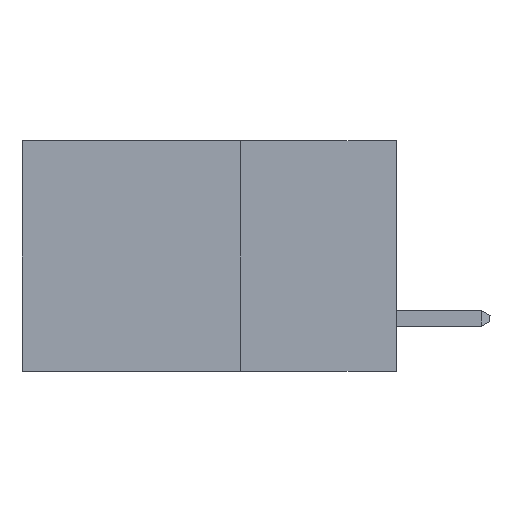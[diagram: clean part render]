
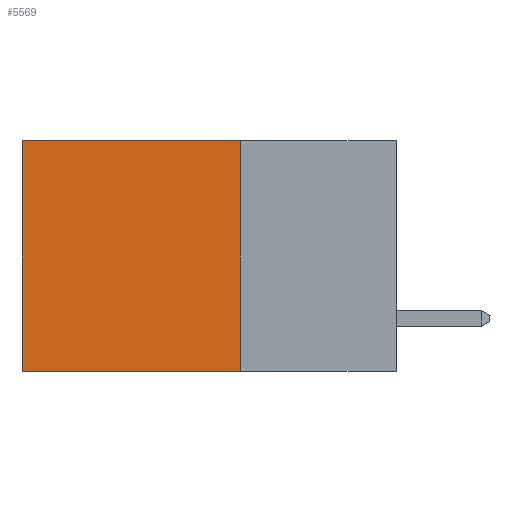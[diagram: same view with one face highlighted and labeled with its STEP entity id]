
A CAD part, left-side view. The second image highlights one B-rep face of the part: STEP entity #5569.
In plain terms, the highlighted planar face has unit normal (-1, 0, 0).
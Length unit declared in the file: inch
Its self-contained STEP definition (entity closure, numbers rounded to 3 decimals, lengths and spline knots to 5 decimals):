
#33 = EDGE_CURVE ( 'NONE', #10502, #3042, #2665, .T. ) ;
#693 = CARTESIAN_POINT ( 'NONE',  ( 0.2615, 0.25, -0.37 ) ) ;
#1177 = DIRECTION ( 'NONE',  ( 0., 0., -1. ) ) ;
#1804 = VECTOR ( 'NONE', #1177, 39.37008 ) ;
#2239 = EDGE_CURVE ( 'NONE', #5415, #3042, #5240, .T. ) ;
#2495 = EDGE_CURVE ( 'NONE', #4620, #10502, #3791, .T. ) ;
#2552 = DIRECTION ( 'NONE',  ( 0., 1., 0. ) ) ;
#2665 = LINE ( 'NONE', #8363, #5552 ) ;
#3042 = VERTEX_POINT ( 'NONE', #3554 ) ;
#3554 = CARTESIAN_POINT ( 'NONE',  ( 0.2615, 0.6, -0.37 ) ) ;
#3639 = CARTESIAN_POINT ( 'NONE',  ( 0.2615, 0.6, 0. ) ) ;
#3664 = ORIENTED_EDGE ( 'NONE', *, *, #33, .F. ) ;
#3739 = DIRECTION ( 'NONE',  ( 0., 0., -1. ) ) ;
#3791 = LINE ( 'NONE', #693, #8138 ) ;
#3816 = VECTOR ( 'NONE', #4326, 39.37008 ) ;
#4326 = DIRECTION ( 'NONE',  ( 0., 1., 0. ) ) ;
#4490 = CARTESIAN_POINT ( 'NONE',  ( 0.2615, 0.6, -0.37 ) ) ;
#4595 = CARTESIAN_POINT ( 'NONE',  ( 0.2615, 0.25, -0.37 ) ) ;
#4620 = VERTEX_POINT ( 'NONE', #9446 ) ;
#5240 = LINE ( 'NONE', #4490, #1804 ) ;
#5415 = VERTEX_POINT ( 'NONE', #3639 ) ;
#5552 = VECTOR ( 'NONE', #2552, 39.37008 ) ;
#5569 = ADVANCED_FACE ( 'NONE', ( #7826 ), #7776, .F. ) ;
#6123 = ORIENTED_EDGE ( 'NONE', *, *, #2495, .F. ) ;
#6519 = AXIS2_PLACEMENT_3D ( 'NONE', #4595, #7943, #3739 ) ;
#6712 = CARTESIAN_POINT ( 'NONE',  ( 0.2615, 0.25, 0. ) ) ;
#6879 = ORIENTED_EDGE ( 'NONE', *, *, #8319, .T. ) ;
#6978 = DIRECTION ( 'NONE',  ( 0., 0., -1. ) ) ;
#7776 = PLANE ( 'NONE',  #6519 ) ;
#7826 = FACE_OUTER_BOUND ( 'NONE', #8968, .T. ) ;
#7943 = DIRECTION ( 'NONE',  ( 1., 0., 0. ) ) ;
#8134 = ORIENTED_EDGE ( 'NONE', *, *, #2239, .T. ) ;
#8138 = VECTOR ( 'NONE', #6978, 39.37008 ) ;
#8319 = EDGE_CURVE ( 'NONE', #4620, #5415, #10102, .T. ) ;
#8363 = CARTESIAN_POINT ( 'NONE',  ( 0.2615, 0.25, -0.37 ) ) ;
#8968 = EDGE_LOOP ( 'NONE', ( #8134, #3664, #6123, #6879 ) ) ;
#9446 = CARTESIAN_POINT ( 'NONE',  ( 0.2615, 0.25, 0. ) ) ;
#10087 = CARTESIAN_POINT ( 'NONE',  ( 0.2615, 0.25, -0.37 ) ) ;
#10102 = LINE ( 'NONE', #6712, #3816 ) ;
#10502 = VERTEX_POINT ( 'NONE', #10087 ) ;
